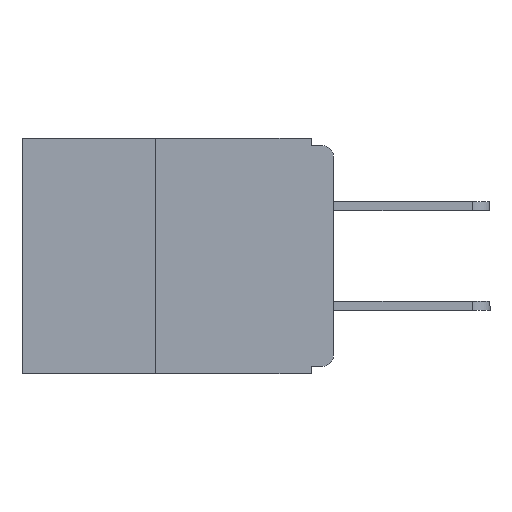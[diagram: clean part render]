
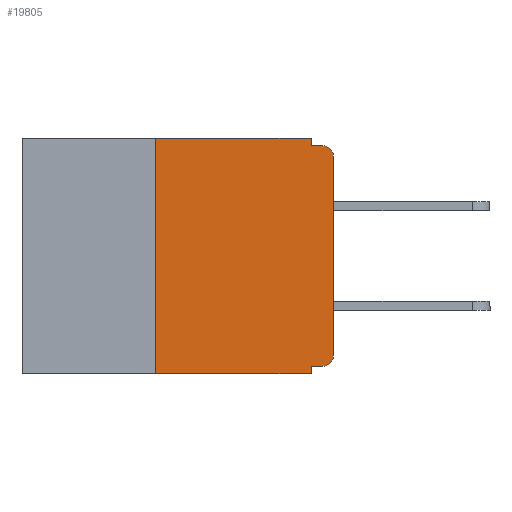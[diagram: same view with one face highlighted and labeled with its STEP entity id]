
A CAD part, left-side view. The second image highlights one B-rep face of the part: STEP entity #19805.
In plain terms, the highlighted planar face has unit normal (-1, 0, 0).
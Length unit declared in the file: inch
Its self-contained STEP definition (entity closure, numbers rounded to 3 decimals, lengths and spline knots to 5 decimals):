
#437 = ORIENTED_EDGE ( 'NONE', *, *, #29249, .T. ) ;
#767 = DIRECTION ( 'NONE',  ( 0., -1., 0. ) ) ;
#812 = DIRECTION ( 'NONE',  ( 1., 0., 0. ) ) ;
#845 = CARTESIAN_POINT ( 'NONE',  ( 0., 0., -0.32 ) ) ;
#907 = DIRECTION ( 'NONE',  ( 0., 1., 0. ) ) ;
#1667 = CARTESIAN_POINT ( 'NONE',  ( 0., 0.031, 0. ) ) ;
#1827 = CARTESIAN_POINT ( 'NONE',  ( 0., 0.031, -0.33 ) ) ;
#1942 = DIRECTION ( 'NONE',  ( 0., 0., 1. ) ) ;
#2268 = VECTOR ( 'NONE', #11472, 39.37008 ) ;
#2883 = EDGE_CURVE ( 'NONE', #9075, #26477, #18987, .T. ) ;
#3110 = DIRECTION ( 'NONE',  ( 0., 0., 1. ) ) ;
#3982 = CARTESIAN_POINT ( 'NONE',  ( 0., 0.015, -0.025 ) ) ;
#5097 = FACE_OUTER_BOUND ( 'NONE', #15007, .T. ) ;
#5306 = CIRCLE ( 'NONE', #23914, 0.015 ) ;
#5380 = VECTOR ( 'NONE', #767, 39.37008 ) ;
#5391 = CARTESIAN_POINT ( 'NONE',  ( 0., 0.031, -0.33 ) ) ;
#5584 = VERTEX_POINT ( 'NONE', #6712 ) ;
#5707 = CARTESIAN_POINT ( 'NONE',  ( 0., 0.031, -0.32 ) ) ;
#5883 = LINE ( 'NONE', #1827, #12074 ) ;
#6139 = VERTEX_POINT ( 'NONE', #16359 ) ;
#6345 = DIRECTION ( 'NONE',  ( 0., 0., -1. ) ) ;
#6712 = CARTESIAN_POINT ( 'NONE',  ( 0., 0., -0.025 ) ) ;
#7893 = VERTEX_POINT ( 'NONE', #19402 ) ;
#7975 = CARTESIAN_POINT ( 'NONE',  ( 0., 0.437, 0. ) ) ;
#8157 = CARTESIAN_POINT ( 'NONE',  ( 0., 0.25, -0.33 ) ) ;
#8571 = CARTESIAN_POINT ( 'NONE',  ( 0., 0.015, -0.305 ) ) ;
#8726 = VERTEX_POINT ( 'NONE', #1667 ) ;
#8788 = LINE ( 'NONE', #7975, #14922 ) ;
#9075 = VERTEX_POINT ( 'NONE', #10141 ) ;
#9902 = EDGE_CURVE ( 'NONE', #26477, #24572, #5883, .T. ) ;
#10141 = CARTESIAN_POINT ( 'NONE',  ( 0., 0.015, -0.32 ) ) ;
#10351 = DIRECTION ( 'NONE',  ( 0., -1., 0. ) ) ;
#10957 = DIRECTION ( 'NONE',  ( 0., 0., -1. ) ) ;
#11472 = DIRECTION ( 'NONE',  ( 0., 0., -1. ) ) ;
#12074 = VECTOR ( 'NONE', #17825, 39.37008 ) ;
#12175 = CARTESIAN_POINT ( 'NONE',  ( 0., 0.437, -0.33 ) ) ;
#12265 = EDGE_CURVE ( 'NONE', #27013, #7893, #21460, .T. ) ;
#13001 = EDGE_CURVE ( 'NONE', #26518, #24572, #17562, .T. ) ;
#13047 = ORIENTED_EDGE ( 'NONE', *, *, #9902, .F. ) ;
#13776 = AXIS2_PLACEMENT_3D ( 'NONE', #3982, #20005, #6345 ) ;
#14552 = ORIENTED_EDGE ( 'NONE', *, *, #22759, .T. ) ;
#14591 = CARTESIAN_POINT ( 'NONE',  ( 0., 0.437, 0. ) ) ;
#14659 = LINE ( 'NONE', #23557, #25136 ) ;
#14773 = VERTEX_POINT ( 'NONE', #27410 ) ;
#14779 = ORIENTED_EDGE ( 'NONE', *, *, #21810, .T. ) ;
#14922 = VECTOR ( 'NONE', #10351, 39.37008 ) ;
#15007 = EDGE_LOOP ( 'NONE', ( #14552, #437, #29086, #24942, #16959, #27890, #28353, #13047, #17839, #14779 ) ) ;
#16009 = EDGE_CURVE ( 'NONE', #26518, #6139, #25431, .T. ) ;
#16359 = CARTESIAN_POINT ( 'NONE',  ( 0., 0.25, 0. ) ) ;
#16797 = DIRECTION ( 'NONE',  ( 0., 0., -1. ) ) ;
#16959 = ORIENTED_EDGE ( 'NONE', *, *, #23442, .F. ) ;
#17392 = CIRCLE ( 'NONE', #13776, 0.015 ) ;
#17562 = LINE ( 'NONE', #12175, #5380 ) ;
#17825 = DIRECTION ( 'NONE',  ( 0., 0., -1. ) ) ;
#17839 = ORIENTED_EDGE ( 'NONE', *, *, #2883, .F. ) ;
#18267 = VECTOR ( 'NONE', #907, 39.37008 ) ;
#18987 = LINE ( 'NONE', #845, #18267 ) ;
#19025 = EDGE_CURVE ( 'NONE', #8726, #27013, #20513, .T. ) ;
#19195 = DIRECTION ( 'NONE',  ( 0., -1., 0. ) ) ;
#19402 = CARTESIAN_POINT ( 'NONE',  ( 0., 0.015, -0.01 ) ) ;
#19404 = VECTOR ( 'NONE', #19195, 39.37008 ) ;
#19805 = ADVANCED_FACE ( 'NONE', ( #5097 ), #27933, .F. ) ;
#20005 = DIRECTION ( 'NONE',  ( -1., 0., 0. ) ) ;
#20391 = CARTESIAN_POINT ( 'NONE',  ( 0., 0.031, 0. ) ) ;
#20513 = LINE ( 'NONE', #20391, #2268 ) ;
#21460 = LINE ( 'NONE', #28039, #19404 ) ;
#21810 = EDGE_CURVE ( 'NONE', #9075, #14773, #5306, .T. ) ;
#22759 = EDGE_CURVE ( 'NONE', #14773, #5584, #14659, .T. ) ;
#23442 = EDGE_CURVE ( 'NONE', #6139, #8726, #8788, .T. ) ;
#23557 = CARTESIAN_POINT ( 'NONE',  ( 0., 0., 0. ) ) ;
#23914 = AXIS2_PLACEMENT_3D ( 'NONE', #8571, #24374, #10957 ) ;
#24374 = DIRECTION ( 'NONE',  ( -1., 0., 0. ) ) ;
#24572 = VERTEX_POINT ( 'NONE', #5391 ) ;
#24741 = VECTOR ( 'NONE', #1942, 39.37008 ) ;
#24815 = AXIS2_PLACEMENT_3D ( 'NONE', #14591, #812, #16797 ) ;
#24942 = ORIENTED_EDGE ( 'NONE', *, *, #19025, .F. ) ;
#25136 = VECTOR ( 'NONE', #3110, 39.37008 ) ;
#25431 = LINE ( 'NONE', #29032, #24741 ) ;
#26477 = VERTEX_POINT ( 'NONE', #5707 ) ;
#26518 = VERTEX_POINT ( 'NONE', #8157 ) ;
#27013 = VERTEX_POINT ( 'NONE', #28012 ) ;
#27410 = CARTESIAN_POINT ( 'NONE',  ( 0., 0., -0.305 ) ) ;
#27890 = ORIENTED_EDGE ( 'NONE', *, *, #16009, .F. ) ;
#27933 = PLANE ( 'NONE',  #24815 ) ;
#28012 = CARTESIAN_POINT ( 'NONE',  ( 0., 0.031, -0.01 ) ) ;
#28039 = CARTESIAN_POINT ( 'NONE',  ( 0., 0., -0.01 ) ) ;
#28353 = ORIENTED_EDGE ( 'NONE', *, *, #13001, .T. ) ;
#29032 = CARTESIAN_POINT ( 'NONE',  ( 0., 0.25, -0.33 ) ) ;
#29086 = ORIENTED_EDGE ( 'NONE', *, *, #12265, .F. ) ;
#29249 = EDGE_CURVE ( 'NONE', #5584, #7893, #17392, .T. ) ;
